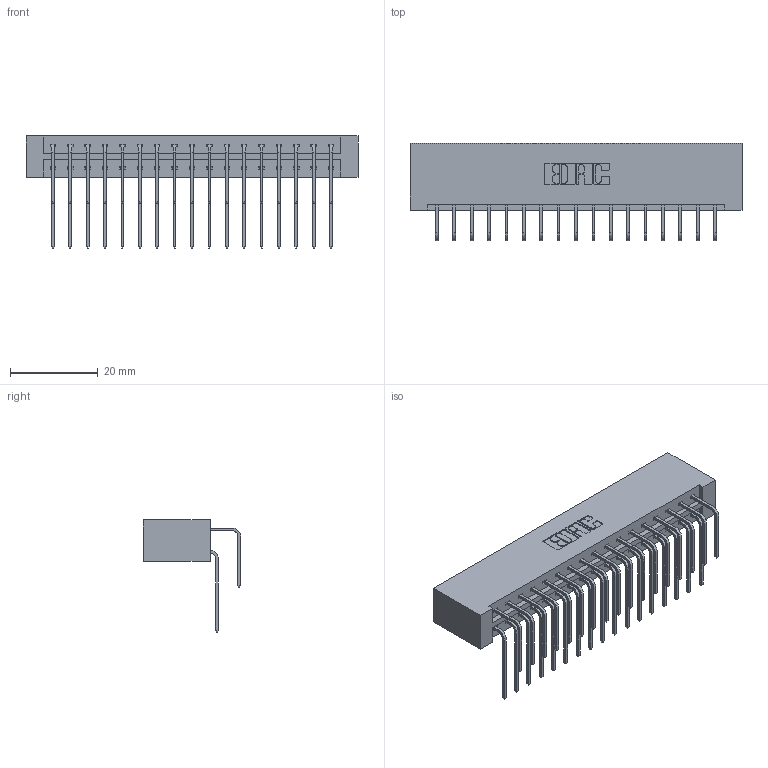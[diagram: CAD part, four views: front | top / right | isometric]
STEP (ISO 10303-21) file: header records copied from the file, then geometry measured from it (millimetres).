
FILE_DESCRIPTION (( 'STEP AP203' ), '1' );
FILE_NAME ('333-034-558-201.STEP', '2018-08-02T22:53:07', ( '' ), ( '' ), 'SwSTEP 2.0', 'SolidWorks 2016', '' );
FILE_SCHEMA (( 'CONFIG_CONTROL_DESIGN' ));
Length unit declared in the file: inch
Products named in the file (4): 345-292-001_558 559 Tail - 1; 345-292-001_558 Tail - 2; 333-034-558-201; 333 Part_Lugless
Assembly tree (35 placements, depth 2):
  333-034-558-201
    333 Part_Lugless
    345-292-001_558 559 Tail - 1  x17
    345-292-001_558 Tail - 2  x17
Bounding box: 75.62 x 22.17 x 25.53 mm (x, y, z)
Volume: 8314.5 mm3; surface area: 10562.5 mm2
Topology: 35 solids, 35 shells, 1942 faces, 5761 edges, 3794 vertices
Faces by surface type: plane 1358, cylinder 584
Entity records: 15677 total; most frequent: CARTESIAN_POINT 2677, ORIENTED_EDGE 2562, DIRECTION 2305, EDGE_CURVE 1281, LINE 1121, VECTOR 1121, VERTEX_POINT 850, AXIS2_PLACEMENT_3D 592
